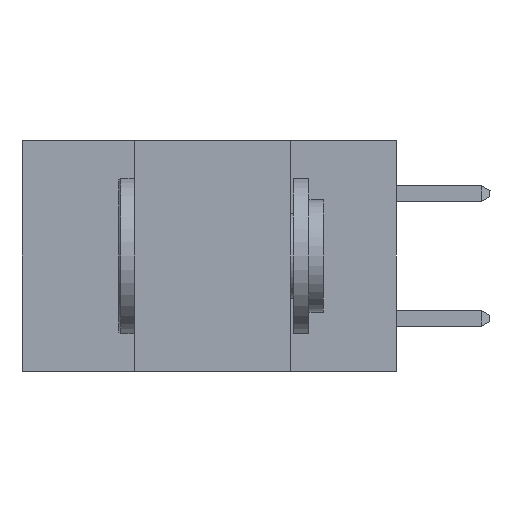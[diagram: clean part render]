
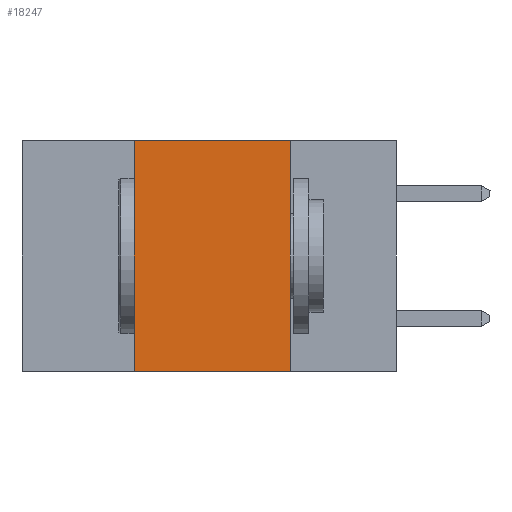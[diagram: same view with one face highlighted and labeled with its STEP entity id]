
A CAD part, left-side view. The second image highlights one B-rep face of the part: STEP entity #18247.
In plain terms, the highlighted planar face has unit normal (-1, 0, 0).
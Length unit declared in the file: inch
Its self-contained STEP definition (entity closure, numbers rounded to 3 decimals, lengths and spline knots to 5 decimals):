
#55 = DIRECTION ( 'NONE',  ( 1., 0., 0. ) ) ;
#695 = CARTESIAN_POINT ( 'NONE',  ( 0., 0.42, 0. ) ) ;
#1230 = VECTOR ( 'NONE', #13274, 39.37008 ) ;
#1874 = VECTOR ( 'NONE', #4354, 39.37008 ) ;
#2423 = LINE ( 'NONE', #21553, #1874 ) ;
#2644 = FACE_OUTER_BOUND ( 'NONE', #14508, .T. ) ;
#3981 = VECTOR ( 'NONE', #21750, 39.37008 ) ;
#4354 = DIRECTION ( 'NONE',  ( 0., 0., -1. ) ) ;
#5692 = ORIENTED_EDGE ( 'NONE', *, *, #10898, .T. ) ;
#7780 = LINE ( 'NONE', #695, #16902 ) ;
#8030 = CARTESIAN_POINT ( 'NONE',  ( 0., 0.6, 0. ) ) ;
#8465 = VERTEX_POINT ( 'NONE', #18435 ) ;
#9178 = LINE ( 'NONE', #8030, #3981 ) ;
#9842 = ORIENTED_EDGE ( 'NONE', *, *, #18635, .F. ) ;
#9973 = ORIENTED_EDGE ( 'NONE', *, *, #13454, .F. ) ;
#10218 = VERTEX_POINT ( 'NONE', #18128 ) ;
#10576 = CARTESIAN_POINT ( 'NONE',  ( 0., 0.6, 0. ) ) ;
#10898 = EDGE_CURVE ( 'NONE', #8465, #10218, #19022, .T. ) ;
#12335 = DIRECTION ( 'NONE',  ( 0., 0., -1. ) ) ;
#12399 = VERTEX_POINT ( 'NONE', #22113 ) ;
#13274 = DIRECTION ( 'NONE',  ( 0., -1., 0. ) ) ;
#13454 = EDGE_CURVE ( 'NONE', #15253, #10218, #2423, .T. ) ;
#14508 = EDGE_LOOP ( 'NONE', ( #9973, #9842, #19102, #5692 ) ) ;
#15209 = AXIS2_PLACEMENT_3D ( 'NONE', #10576, #55, #12335 ) ;
#15253 = VERTEX_POINT ( 'NONE', #16362 ) ;
#15896 = EDGE_CURVE ( 'NONE', #8465, #12399, #7780, .T. ) ;
#16257 = DIRECTION ( 'NONE',  ( 0., 0., 1. ) ) ;
#16362 = CARTESIAN_POINT ( 'NONE',  ( 0., 0.17, 0. ) ) ;
#16902 = VECTOR ( 'NONE', #16257, 39.37008 ) ;
#18128 = CARTESIAN_POINT ( 'NONE',  ( 0., 0.17, -0.37 ) ) ;
#18247 = ADVANCED_FACE ( 'NONE', ( #2644 ), #19035, .F. ) ;
#18340 = CARTESIAN_POINT ( 'NONE',  ( 0., 0.6, -0.37 ) ) ;
#18435 = CARTESIAN_POINT ( 'NONE',  ( 0., 0.42, -0.37 ) ) ;
#18635 = EDGE_CURVE ( 'NONE', #12399, #15253, #9178, .T. ) ;
#19022 = LINE ( 'NONE', #18340, #1230 ) ;
#19035 = PLANE ( 'NONE',  #15209 ) ;
#19102 = ORIENTED_EDGE ( 'NONE', *, *, #15896, .F. ) ;
#21553 = CARTESIAN_POINT ( 'NONE',  ( 0., 0.17, 0. ) ) ;
#21750 = DIRECTION ( 'NONE',  ( 0., -1., 0. ) ) ;
#22113 = CARTESIAN_POINT ( 'NONE',  ( 0., 0.42, 0. ) ) ;
